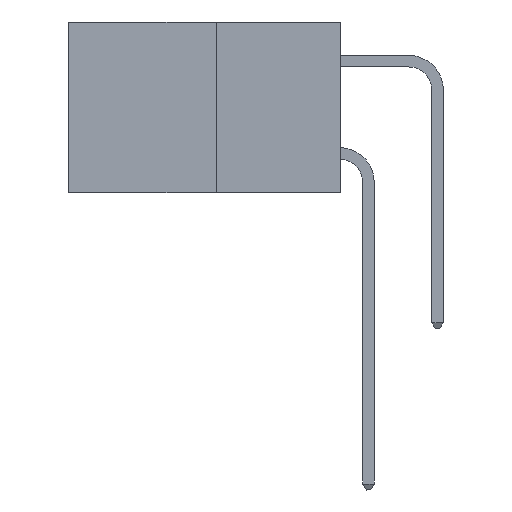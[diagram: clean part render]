
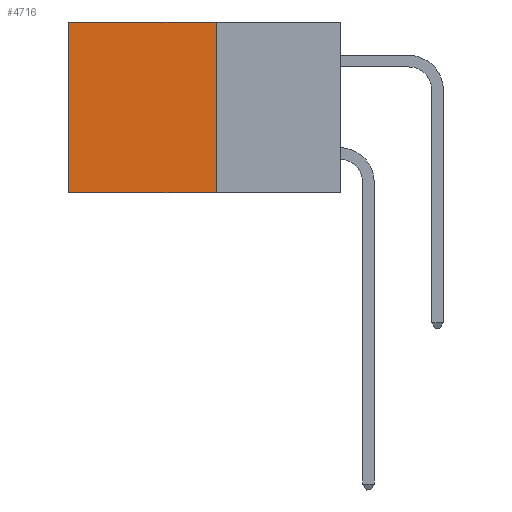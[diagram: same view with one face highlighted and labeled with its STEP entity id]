
A CAD part, left-side view. The second image highlights one B-rep face of the part: STEP entity #4716.
In plain terms, the highlighted planar face has unit normal (-1, 0, 0).
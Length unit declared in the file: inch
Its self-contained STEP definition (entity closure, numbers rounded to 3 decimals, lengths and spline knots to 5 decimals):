
#535 = CARTESIAN_POINT ( 'NONE',  ( 0.277, 0.27, -0.37 ) ) ;
#619 = FACE_OUTER_BOUND ( 'NONE', #7015, .T. ) ;
#685 = DIRECTION ( 'NONE',  ( 0., 0., -1. ) ) ;
#724 = EDGE_CURVE ( 'NONE', #7000, #5777, #1193, .T. ) ;
#914 = LINE ( 'NONE', #2043, #3030 ) ;
#1082 = DIRECTION ( 'NONE',  ( 0., 1., 0. ) ) ;
#1193 = LINE ( 'NONE', #4732, #5234 ) ;
#1577 = CARTESIAN_POINT ( 'NONE',  ( 0.277, 0.27, -0.37 ) ) ;
#1761 = CARTESIAN_POINT ( 'NONE',  ( 0.277, 0.27, 0. ) ) ;
#2043 = CARTESIAN_POINT ( 'NONE',  ( 0.277, 0.27, -0.37 ) ) ;
#3030 = VECTOR ( 'NONE', #5040, 39.37008 ) ;
#3088 = DIRECTION ( 'NONE',  ( 0., 0., -1. ) ) ;
#3537 = DIRECTION ( 'NONE',  ( 0., 0., -1. ) ) ;
#4716 = ADVANCED_FACE ( 'NONE', ( #619 ), #4957, .F. ) ;
#4732 = CARTESIAN_POINT ( 'NONE',  ( 0.277, 0.59, -0.37 ) ) ;
#4875 = VECTOR ( 'NONE', #685, 39.37008 ) ;
#4957 = PLANE ( 'NONE',  #9600 ) ;
#5040 = DIRECTION ( 'NONE',  ( 0., 1., 0. ) ) ;
#5047 = VECTOR ( 'NONE', #1082, 39.37008 ) ;
#5185 = EDGE_CURVE ( 'NONE', #6588, #5777, #914, .T. ) ;
#5234 = VECTOR ( 'NONE', #3088, 39.37008 ) ;
#5777 = VERTEX_POINT ( 'NONE', #9450 ) ;
#5984 = CARTESIAN_POINT ( 'NONE',  ( 0.277, 0.27, -0.37 ) ) ;
#6364 = CARTESIAN_POINT ( 'NONE',  ( 0.277, 0.27, 0. ) ) ;
#6474 = EDGE_CURVE ( 'NONE', #10109, #7000, #6982, .T. ) ;
#6477 = ORIENTED_EDGE ( 'NONE', *, *, #6474, .T. ) ;
#6588 = VERTEX_POINT ( 'NONE', #535 ) ;
#6982 = LINE ( 'NONE', #1761, #5047 ) ;
#7000 = VERTEX_POINT ( 'NONE', #9817 ) ;
#7015 = EDGE_LOOP ( 'NONE', ( #9734, #9693, #8784, #6477 ) ) ;
#7309 = DIRECTION ( 'NONE',  ( 1., 0., 0. ) ) ;
#8784 = ORIENTED_EDGE ( 'NONE', *, *, #9097, .F. ) ;
#9097 = EDGE_CURVE ( 'NONE', #10109, #6588, #9208, .T. ) ;
#9208 = LINE ( 'NONE', #1577, #4875 ) ;
#9450 = CARTESIAN_POINT ( 'NONE',  ( 0.277, 0.59, -0.37 ) ) ;
#9600 = AXIS2_PLACEMENT_3D ( 'NONE', #5984, #7309, #3537 ) ;
#9693 = ORIENTED_EDGE ( 'NONE', *, *, #5185, .F. ) ;
#9734 = ORIENTED_EDGE ( 'NONE', *, *, #724, .T. ) ;
#9817 = CARTESIAN_POINT ( 'NONE',  ( 0.277, 0.59, 0. ) ) ;
#10109 = VERTEX_POINT ( 'NONE', #6364 ) ;
